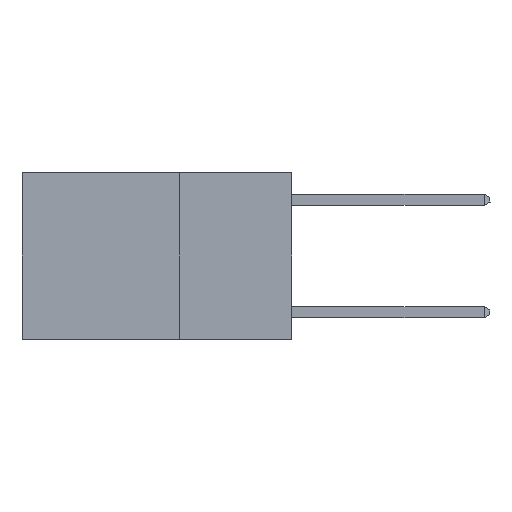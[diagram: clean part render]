
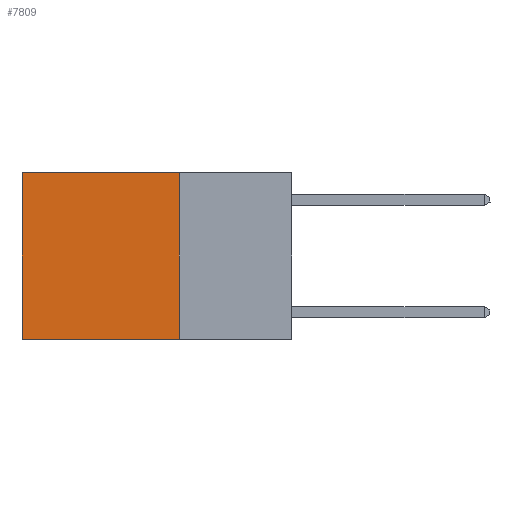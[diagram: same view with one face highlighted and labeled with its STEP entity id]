
A CAD part, left-side view. The second image highlights one B-rep face of the part: STEP entity #7809.
In plain terms, the highlighted planar face has unit normal (-1, 0, 0).
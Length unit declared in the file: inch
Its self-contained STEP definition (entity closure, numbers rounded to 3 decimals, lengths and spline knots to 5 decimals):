
#156 = CARTESIAN_POINT ( 'NONE',  ( 0.2625, 0.6, 0. ) ) ;
#2008 = CARTESIAN_POINT ( 'NONE',  ( 0.2625, 0.6, 0. ) ) ;
#3077 = LINE ( 'NONE', #12029, #10060 ) ;
#3199 = VECTOR ( 'NONE', #17756, 39.37008 ) ;
#3721 = CARTESIAN_POINT ( 'NONE',  ( 0.2625, 0.25, 0. ) ) ;
#4107 = EDGE_CURVE ( 'NONE', #17952, #17381, #7115, .T. ) ;
#4587 = VERTEX_POINT ( 'NONE', #2008 ) ;
#5122 = ORIENTED_EDGE ( 'NONE', *, *, #7599, .T. ) ;
#5139 = ORIENTED_EDGE ( 'NONE', *, *, #14704, .F. ) ;
#5150 = DIRECTION ( 'NONE',  ( 0., 0., -1. ) ) ;
#5151 = ORIENTED_EDGE ( 'NONE', *, *, #4107, .F. ) ;
#5153 = ORIENTED_EDGE ( 'NONE', *, *, #8022, .T. ) ;
#5651 = VECTOR ( 'NONE', #16986, 39.37008 ) ;
#6563 = DIRECTION ( 'NONE',  ( 0., 1., 0. ) ) ;
#7115 = LINE ( 'NONE', #8261, #13940 ) ;
#7554 = CARTESIAN_POINT ( 'NONE',  ( 0.2625, 0.25, -0.37 ) ) ;
#7599 = EDGE_CURVE ( 'NONE', #4587, #9413, #9345, .T. ) ;
#7809 = ADVANCED_FACE ( 'NONE', ( #13551 ), #12005, .F. ) ;
#8022 = EDGE_CURVE ( 'NONE', #17952, #4587, #14193, .T. ) ;
#8261 = CARTESIAN_POINT ( 'NONE',  ( 0.2625, 0.25, 0. ) ) ;
#9345 = LINE ( 'NONE', #156, #5651 ) ;
#9413 = VERTEX_POINT ( 'NONE', #10600 ) ;
#9629 = DIRECTION ( 'NONE',  ( 0., 0., -1. ) ) ;
#10060 = VECTOR ( 'NONE', #6563, 39.37008 ) ;
#10600 = CARTESIAN_POINT ( 'NONE',  ( 0.2625, 0.6, -0.37 ) ) ;
#12005 = PLANE ( 'NONE',  #12316 ) ;
#12029 = CARTESIAN_POINT ( 'NONE',  ( 0.2625, 0.25, -0.37 ) ) ;
#12316 = AXIS2_PLACEMENT_3D ( 'NONE', #3721, #13347, #5150 ) ;
#12548 = EDGE_LOOP ( 'NONE', ( #5122, #5139, #5151, #5153 ) ) ;
#13347 = DIRECTION ( 'NONE',  ( 1., 0., 0. ) ) ;
#13413 = CARTESIAN_POINT ( 'NONE',  ( 0.2625, 0.25, 0. ) ) ;
#13551 = FACE_OUTER_BOUND ( 'NONE', #12548, .T. ) ;
#13940 = VECTOR ( 'NONE', #9629, 39.37008 ) ;
#14193 = LINE ( 'NONE', #16399, #3199 ) ;
#14704 = EDGE_CURVE ( 'NONE', #17381, #9413, #3077, .T. ) ;
#16399 = CARTESIAN_POINT ( 'NONE',  ( 0.2625, 0.25, 0. ) ) ;
#16986 = DIRECTION ( 'NONE',  ( 0., 0., -1. ) ) ;
#17381 = VERTEX_POINT ( 'NONE', #7554 ) ;
#17756 = DIRECTION ( 'NONE',  ( 0., 1., 0. ) ) ;
#17952 = VERTEX_POINT ( 'NONE', #13413 ) ;
